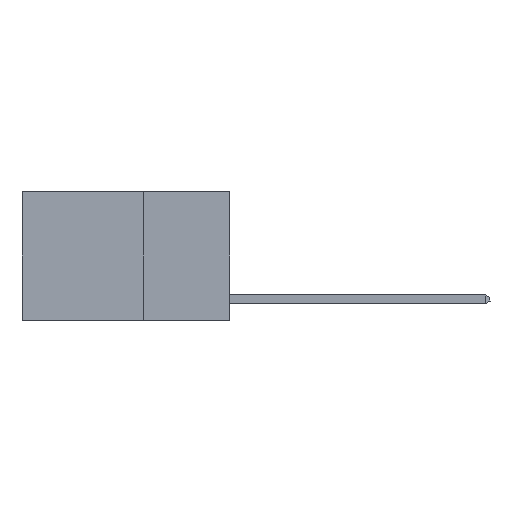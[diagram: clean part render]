
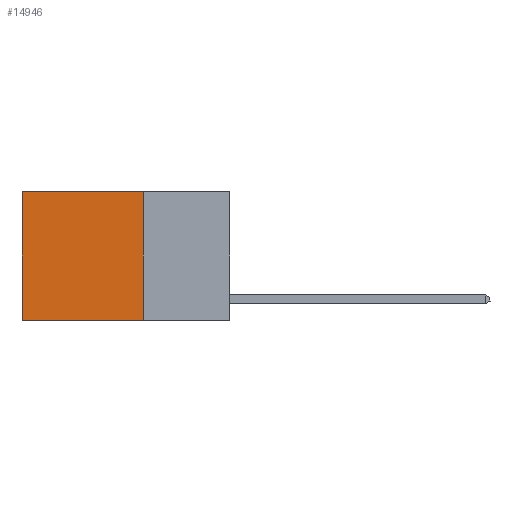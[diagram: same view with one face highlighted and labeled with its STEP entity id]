
A CAD part, left-side view. The second image highlights one B-rep face of the part: STEP entity #14946.
In plain terms, the highlighted planar face has unit normal (-1, 0, 0).
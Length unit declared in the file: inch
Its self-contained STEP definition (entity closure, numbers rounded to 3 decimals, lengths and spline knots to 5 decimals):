
#502 = CARTESIAN_POINT ( 'NONE',  ( 0.2625, 0.25, 0. ) ) ;
#1554 = ORIENTED_EDGE ( 'NONE', *, *, #6426, .T. ) ;
#2003 = EDGE_CURVE ( 'NONE', #2921, #18297, #10989, .T. ) ;
#2404 = VECTOR ( 'NONE', #7004, 39.37008 ) ;
#2921 = VERTEX_POINT ( 'NONE', #7606 ) ;
#3034 = DIRECTION ( 'NONE',  ( 0., 0., -1. ) ) ;
#3812 = CARTESIAN_POINT ( 'NONE',  ( 0.2625, 0.25, -0.37 ) ) ;
#4103 = CARTESIAN_POINT ( 'NONE',  ( 0.2625, 0.6, -0.37 ) ) ;
#5054 = FACE_OUTER_BOUND ( 'NONE', #14491, .T. ) ;
#5477 = ORIENTED_EDGE ( 'NONE', *, *, #11191, .T. ) ;
#6426 = EDGE_CURVE ( 'NONE', #2921, #8679, #12793, .T. ) ;
#7004 = DIRECTION ( 'NONE',  ( 0., 0., -1. ) ) ;
#7385 = CARTESIAN_POINT ( 'NONE',  ( 0.2625, 0.25, 0. ) ) ;
#7500 = EDGE_CURVE ( 'NONE', #18297, #9271, #15993, .T. ) ;
#7606 = CARTESIAN_POINT ( 'NONE',  ( 0.2625, 0.25, 0. ) ) ;
#8301 = CARTESIAN_POINT ( 'NONE',  ( 0.2625, 0.25, -0.37 ) ) ;
#8551 = VECTOR ( 'NONE', #14893, 39.37008 ) ;
#8679 = VERTEX_POINT ( 'NONE', #14668 ) ;
#9018 = DIRECTION ( 'NONE',  ( 0., 0., -1. ) ) ;
#9271 = VERTEX_POINT ( 'NONE', #4103 ) ;
#9893 = DIRECTION ( 'NONE',  ( 0., 1., 0. ) ) ;
#10989 = LINE ( 'NONE', #502, #2404 ) ;
#11191 = EDGE_CURVE ( 'NONE', #8679, #9271, #19270, .T. ) ;
#12161 = ORIENTED_EDGE ( 'NONE', *, *, #7500, .F. ) ;
#12793 = LINE ( 'NONE', #19564, #8551 ) ;
#14491 = EDGE_LOOP ( 'NONE', ( #5477, #12161, #17966, #1554 ) ) ;
#14668 = CARTESIAN_POINT ( 'NONE',  ( 0.2625, 0.6, 0. ) ) ;
#14893 = DIRECTION ( 'NONE',  ( 0., 1., 0. ) ) ;
#14946 = ADVANCED_FACE ( 'NONE', ( #5054 ), #15357, .F. ) ;
#15357 = PLANE ( 'NONE',  #17432 ) ;
#15482 = VECTOR ( 'NONE', #9893, 39.37008 ) ;
#15872 = CARTESIAN_POINT ( 'NONE',  ( 0.2625, 0.6, 0. ) ) ;
#15993 = LINE ( 'NONE', #8301, #15482 ) ;
#17432 = AXIS2_PLACEMENT_3D ( 'NONE', #7385, #18534, #9018 ) ;
#17966 = ORIENTED_EDGE ( 'NONE', *, *, #2003, .F. ) ;
#18297 = VERTEX_POINT ( 'NONE', #3812 ) ;
#18534 = DIRECTION ( 'NONE',  ( 1., 0., 0. ) ) ;
#19270 = LINE ( 'NONE', #15872, #20218 ) ;
#19564 = CARTESIAN_POINT ( 'NONE',  ( 0.2625, 0.25, 0. ) ) ;
#20218 = VECTOR ( 'NONE', #3034, 39.37008 ) ;
